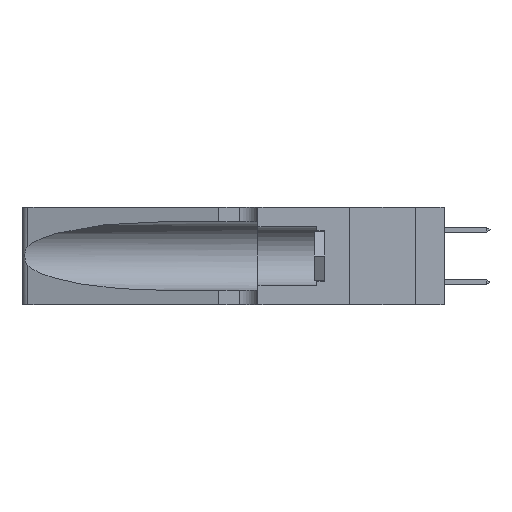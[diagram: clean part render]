
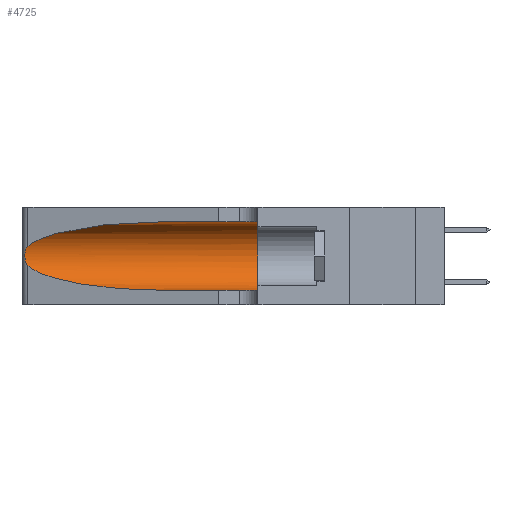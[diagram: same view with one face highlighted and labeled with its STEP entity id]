
A CAD part, left-side view. The second image highlights one B-rep face of the part: STEP entity #4725.
In plain terms, the highlighted cylindrical face has radius 3.308 mm (diameter 6.617 mm), a partial arc.
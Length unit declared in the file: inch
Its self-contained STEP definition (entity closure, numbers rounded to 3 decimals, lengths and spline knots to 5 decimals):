
#684 = CARTESIAN_POINT ( 'NONE',  ( 0.1305, 0.35, 0.05475 ) ) ;
#795 = B_SPLINE_CURVE_WITH_KNOTS ( 'NONE', 3,
 ( #13358, #25875, #17835, #26158, #3001, #13635, #13727, #3184, #1243, #19765, #19944, #23825, #17926, #7539 ),
 .UNSPECIFIED., .F., .F.,
 ( 4, 2, 2, 2, 2, 2, 4 ),
 ( 0., 0.00027, 0.00053, 0.00107, 0.0016, 0.00187, 0.00214 ),
 .UNSPECIFIED. ) ;
#1219 = CARTESIAN_POINT ( 'NONE',  ( 0.25487, 1.22718, 0.14631 ) ) ;
#1243 = CARTESIAN_POINT ( 'NONE',  ( 0.26017, 1.23833, 0.17102 ) ) ;
#1356 = DIRECTION ( 'NONE',  ( 0., -1., 0. ) ) ;
#1703 = CARTESIAN_POINT ( 'NONE',  ( 0.1305, 1.61858, 0.31525 ) ) ;
#2302 = FACE_OUTER_BOUND ( 'NONE', #18898, .T. ) ;
#3001 = CARTESIAN_POINT ( 'NONE',  ( 0.25854, 1.2359, 0.20912 ) ) ;
#3184 = CARTESIAN_POINT ( 'NONE',  ( 0.26075, 1.23896, 0.178 ) ) ;
#3337 = LINE ( 'NONE', #13841, #13746 ) ;
#3655 = CARTESIAN_POINT ( 'NONE',  ( 0.25487, 1.22718, 0.22369 ) ) ;
#4046 = DIRECTION ( 'NONE',  ( 0., 0., -1. ) ) ;
#4490 =( BOUNDED_CURVE ( )  B_SPLINE_CURVE ( 3, ( #10782, #8868, #8780, #23458 ),
 .UNSPECIFIED., .F., .T. ) 
 B_SPLINE_CURVE_WITH_KNOTS ( ( 4, 4 ),
 ( 1.5708, 2.84003 ),
 .UNSPECIFIED. ) 
 CURVE ( )  GEOMETRIC_REPRESENTATION_ITEM ( )  RATIONAL_B_SPLINE_CURVE ( ( 1., 0.87, 0.87, 1. ) ) 
 REPRESENTATION_ITEM ( '' )  );
#4662 = VERTEX_POINT ( 'NONE', #3655 ) ;
#4725 = ADVANCED_FACE ( 'NONE', ( #2302 ), #18272, .F. ) ;
#5004 = CARTESIAN_POINT ( 'NONE',  ( 0.25487, 1.22718, 0.14631 ) ) ;
#5726 = CARTESIAN_POINT ( 'NONE',  ( 0.1305, 0.72297, 0.31525 ) ) ;
#6535 = AXIS2_PLACEMENT_3D ( 'NONE', #26372, #18137, #19982 ) ;
#7060 = VERTEX_POINT ( 'NONE', #684 ) ;
#7520 = AXIS2_PLACEMENT_3D ( 'NONE', #18521, #20262, #4046 ) ;
#7539 = CARTESIAN_POINT ( 'NONE',  ( 0.25487, 1.22718, 0.14631 ) ) ;
#8676 = DIRECTION ( 'NONE',  ( 0., -1., 0. ) ) ;
#8780 = CARTESIAN_POINT ( 'NONE',  ( 0.2373, 1.15595, 0.28018 ) ) ;
#8868 = CARTESIAN_POINT ( 'NONE',  ( 0.18966, 0.96281, 0.31525 ) ) ;
#9005 = VERTEX_POINT ( 'NONE', #17341 ) ;
#10517 = CARTESIAN_POINT ( 'NONE',  ( 0.1305, 0.35, 0.31525 ) ) ;
#10782 = CARTESIAN_POINT ( 'NONE',  ( 0.1305, 0.72297, 0.31525 ) ) ;
#12143 =( BOUNDED_CURVE ( )  B_SPLINE_CURVE ( 3, ( #1219, #17806, #25934, #21815 ),
 .UNSPECIFIED., .F., .F. ) 
 B_SPLINE_CURVE_WITH_KNOTS ( ( 4, 4 ),
 ( 3.44316, 4.71239 ),
 .UNSPECIFIED. ) 
 CURVE ( )  GEOMETRIC_REPRESENTATION_ITEM ( )  RATIONAL_B_SPLINE_CURVE ( ( 1., 0.87, 0.87, 1. ) ) 
 REPRESENTATION_ITEM ( '' )  );
#12527 = ORIENTED_EDGE ( 'NONE', *, *, #13146, .F. ) ;
#13146 = EDGE_CURVE ( 'NONE', #26922, #23945, #16928, .T. ) ;
#13358 = CARTESIAN_POINT ( 'NONE',  ( 0.25487, 1.22718, 0.22369 ) ) ;
#13635 = CARTESIAN_POINT ( 'NONE',  ( 0.26018, 1.23835, 0.19895 ) ) ;
#13727 = CARTESIAN_POINT ( 'NONE',  ( 0.26075, 1.23896, 0.19203 ) ) ;
#13746 = VECTOR ( 'NONE', #1356, 39.37008 ) ;
#13841 = CARTESIAN_POINT ( 'NONE',  ( 0.1305, 1.61858, 0.05475 ) ) ;
#14764 = EDGE_CURVE ( 'NONE', #23945, #7060, #17071, .T. ) ;
#15577 = EDGE_CURVE ( 'NONE', #9005, #7060, #3337, .T. ) ;
#16928 = LINE ( 'NONE', #1703, #19565 ) ;
#17071 = CIRCLE ( 'NONE', #6535, 0.13025 ) ;
#17341 = CARTESIAN_POINT ( 'NONE',  ( 0.1305, 0.72297, 0.05475 ) ) ;
#17806 = CARTESIAN_POINT ( 'NONE',  ( 0.2373, 1.15595, 0.08982 ) ) ;
#17835 = CARTESIAN_POINT ( 'NONE',  ( 0.25639, 1.23184, 0.21858 ) ) ;
#17926 = CARTESIAN_POINT ( 'NONE',  ( 0.25555, 1.22993, 0.14849 ) ) ;
#18137 = DIRECTION ( 'NONE',  ( 0., 1., 0. ) ) ;
#18188 = ORIENTED_EDGE ( 'NONE', *, *, #18567, .T. ) ;
#18272 = CYLINDRICAL_SURFACE ( 'NONE', #7520, 0.13025 ) ;
#18521 = CARTESIAN_POINT ( 'NONE',  ( 0.1305, 1.61858, 0.185 ) ) ;
#18567 = EDGE_CURVE ( 'NONE', #26922, #4662, #4490, .T. ) ;
#18898 = EDGE_LOOP ( 'NONE', ( #18188, #22654, #21000, #21643, #26581, #12527 ) ) ;
#19565 = VECTOR ( 'NONE', #8676, 39.37008 ) ;
#19765 = CARTESIAN_POINT ( 'NONE',  ( 0.25856, 1.23593, 0.16098 ) ) ;
#19944 = CARTESIAN_POINT ( 'NONE',  ( 0.25789, 1.23486, 0.15765 ) ) ;
#19982 = DIRECTION ( 'NONE',  ( 0., 0., 1. ) ) ;
#20262 = DIRECTION ( 'NONE',  ( 0., -1., 0. ) ) ;
#21000 = ORIENTED_EDGE ( 'NONE', *, *, #24798, .T. ) ;
#21643 = ORIENTED_EDGE ( 'NONE', *, *, #15577, .T. ) ;
#21815 = CARTESIAN_POINT ( 'NONE',  ( 0.1305, 0.72297, 0.05475 ) ) ;
#22233 = EDGE_CURVE ( 'NONE', #4662, #24193, #795, .T. ) ;
#22654 = ORIENTED_EDGE ( 'NONE', *, *, #22233, .T. ) ;
#23458 = CARTESIAN_POINT ( 'NONE',  ( 0.25487, 1.22718, 0.22369 ) ) ;
#23825 = CARTESIAN_POINT ( 'NONE',  ( 0.25639, 1.23186, 0.15144 ) ) ;
#23945 = VERTEX_POINT ( 'NONE', #10517 ) ;
#24193 = VERTEX_POINT ( 'NONE', #5004 ) ;
#24798 = EDGE_CURVE ( 'NONE', #24193, #9005, #12143, .T. ) ;
#25875 = CARTESIAN_POINT ( 'NONE',  ( 0.25555, 1.22994, 0.2215 ) ) ;
#25934 = CARTESIAN_POINT ( 'NONE',  ( 0.18966, 0.96281, 0.05475 ) ) ;
#26158 = CARTESIAN_POINT ( 'NONE',  ( 0.25787, 1.23484, 0.2124 ) ) ;
#26372 = CARTESIAN_POINT ( 'NONE',  ( 0.1305, 0.35, 0.185 ) ) ;
#26581 = ORIENTED_EDGE ( 'NONE', *, *, #14764, .F. ) ;
#26922 = VERTEX_POINT ( 'NONE', #5726 ) ;
